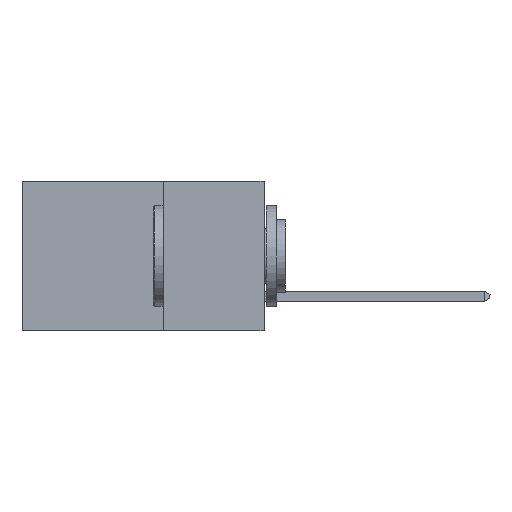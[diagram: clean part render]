
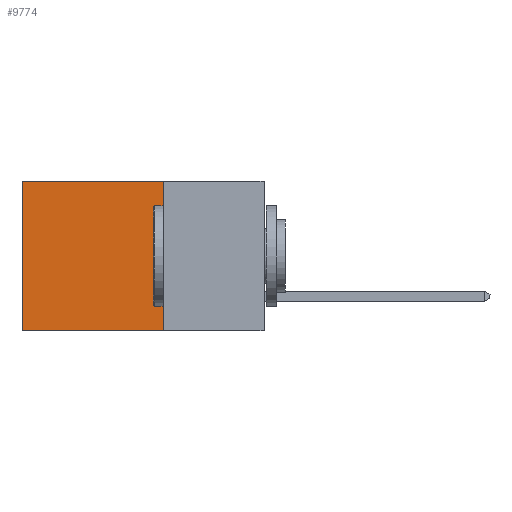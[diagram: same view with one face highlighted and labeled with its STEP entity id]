
A CAD part, left-side view. The second image highlights one B-rep face of the part: STEP entity #9774.
In plain terms, the highlighted planar face has unit normal (-1, 0, 0).
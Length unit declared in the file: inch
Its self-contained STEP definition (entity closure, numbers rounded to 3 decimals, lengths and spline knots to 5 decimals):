
#346 = DIRECTION ( 'NONE',  ( 0., 0., -1. ) ) ;
#394 = PLANE ( 'NONE',  #2450 ) ;
#696 = CARTESIAN_POINT ( 'NONE',  ( 0.2615, 0.25, 0. ) ) ;
#810 = ORIENTED_EDGE ( 'NONE', *, *, #1015, .F. ) ;
#949 = EDGE_CURVE ( 'NONE', #9902, #5324, #4328, .T. ) ;
#1015 = EDGE_CURVE ( 'NONE', #3982, #4612, #5029, .T. ) ;
#1601 = VECTOR ( 'NONE', #3488, 39.37008 ) ;
#1865 = EDGE_LOOP ( 'NONE', ( #7810, #5130, #810, #5056 ) ) ;
#2142 = DIRECTION ( 'NONE',  ( 0., 1., 0. ) ) ;
#2182 = CARTESIAN_POINT ( 'NONE',  ( 0.2615, 0.6, 0. ) ) ;
#2450 = AXIS2_PLACEMENT_3D ( 'NONE', #4232, #7309, #8129 ) ;
#2524 = VECTOR ( 'NONE', #4519, 39.37008 ) ;
#2892 = FACE_OUTER_BOUND ( 'NONE', #1865, .T. ) ;
#2981 = LINE ( 'NONE', #696, #2524 ) ;
#3008 = CARTESIAN_POINT ( 'NONE',  ( 0.2615, 0.25, 0. ) ) ;
#3122 = CARTESIAN_POINT ( 'NONE',  ( 0.2615, 0.6, -0.37 ) ) ;
#3432 = CARTESIAN_POINT ( 'NONE',  ( 0.2615, 0.25, -0.37 ) ) ;
#3488 = DIRECTION ( 'NONE',  ( 0., 0., -1. ) ) ;
#3982 = VERTEX_POINT ( 'NONE', #3008 ) ;
#4232 = CARTESIAN_POINT ( 'NONE',  ( 0.2615, 0.25, -0.37 ) ) ;
#4298 = EDGE_CURVE ( 'NONE', #3982, #9902, #2981, .T. ) ;
#4328 = LINE ( 'NONE', #6599, #1601 ) ;
#4519 = DIRECTION ( 'NONE',  ( 0., 1., 0. ) ) ;
#4612 = VERTEX_POINT ( 'NONE', #3432 ) ;
#5029 = LINE ( 'NONE', #5842, #9619 ) ;
#5056 = ORIENTED_EDGE ( 'NONE', *, *, #4298, .T. ) ;
#5130 = ORIENTED_EDGE ( 'NONE', *, *, #6939, .F. ) ;
#5190 = CARTESIAN_POINT ( 'NONE',  ( 0.2615, 0.25, -0.37 ) ) ;
#5324 = VERTEX_POINT ( 'NONE', #3122 ) ;
#5842 = CARTESIAN_POINT ( 'NONE',  ( 0.2615, 0.25, -0.37 ) ) ;
#6158 = LINE ( 'NONE', #5190, #8801 ) ;
#6599 = CARTESIAN_POINT ( 'NONE',  ( 0.2615, 0.6, -0.37 ) ) ;
#6939 = EDGE_CURVE ( 'NONE', #4612, #5324, #6158, .T. ) ;
#7309 = DIRECTION ( 'NONE',  ( 1., 0., 0. ) ) ;
#7810 = ORIENTED_EDGE ( 'NONE', *, *, #949, .T. ) ;
#8129 = DIRECTION ( 'NONE',  ( 0., 0., -1. ) ) ;
#8801 = VECTOR ( 'NONE', #2142, 39.37008 ) ;
#9619 = VECTOR ( 'NONE', #346, 39.37008 ) ;
#9774 = ADVANCED_FACE ( 'NONE', ( #2892 ), #394, .F. ) ;
#9902 = VERTEX_POINT ( 'NONE', #2182 ) ;
